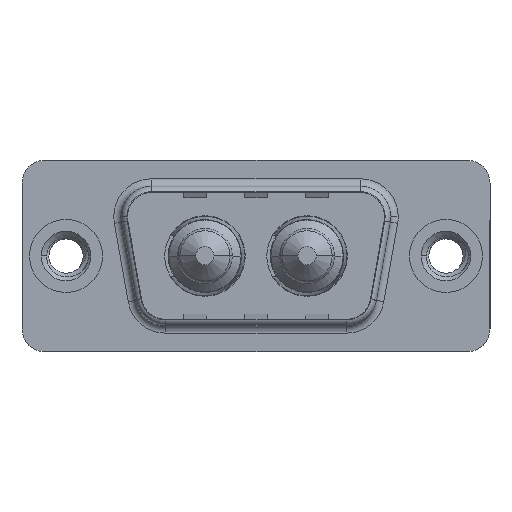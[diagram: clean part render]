
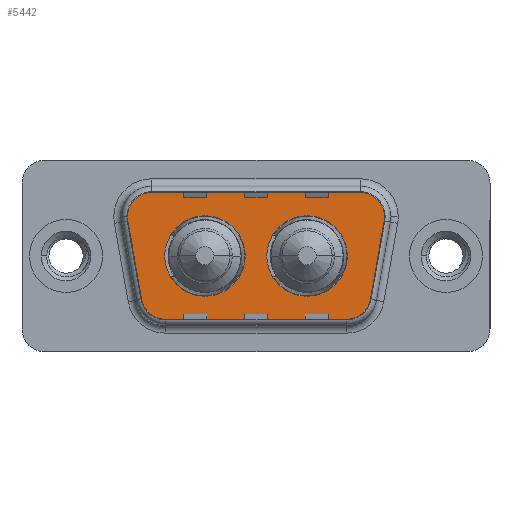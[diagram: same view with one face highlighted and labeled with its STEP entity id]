
A CAD part, top view. The second image highlights one B-rep face of the part: STEP entity #5442.
In plain terms, the highlighted planar face has unit normal (0, 0, 1).
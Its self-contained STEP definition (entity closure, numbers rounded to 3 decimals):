
#39 = CARTESIAN_POINT ( 'NONE',  ( 11.79, 0., 0. ) ) ;
#186 = CARTESIAN_POINT ( 'NONE',  ( 3.466, 2.553, 0. ) ) ;
#323 = EDGE_CURVE ( 'NONE', #8143, #1185, #8012, .T. ) ;
#445 = CARTESIAN_POINT ( 'NONE',  ( 9.14, 0., 0. ) ) ;
#573 = DIRECTION ( 'NONE',  ( 1., 0., 0. ) ) ;
#593 = DIRECTION ( 'NONE',  ( 1., 0., 0. ) ) ;
#618 = DIRECTION ( 'NONE',  ( 1., 0., 0. ) ) ;
#654 = ORIENTED_EDGE ( 'NONE', *, *, #10079, .T. ) ;
#701 = VERTEX_POINT ( 'NONE', #6546 ) ;
#767 = CARTESIAN_POINT ( 'NONE',  ( 21.534, 2.553, 0. ) ) ;
#799 = CIRCLE ( 'NONE', #5250, 2. ) ;
#1023 = EDGE_CURVE ( 'NONE', #1185, #701, #5825, .T. ) ;
#1087 = AXIS2_PLACEMENT_3D ( 'NONE', #2434, #7390, #7545 ) ;
#1137 = EDGE_CURVE ( 'NONE', #2600, #4111, #9660, .T. ) ;
#1185 = VERTEX_POINT ( 'NONE', #8233 ) ;
#1214 = CIRCLE ( 'NONE', #4423, 2.65 ) ;
#1359 = DIRECTION ( 'NONE',  ( 1., 0., 0. ) ) ;
#1370 = AXIS2_PLACEMENT_3D ( 'NONE', #445, #6747, #1359 ) ;
#1387 = FACE_OUTER_BOUND ( 'NONE', #9283, .T. ) ;
#1562 = CARTESIAN_POINT ( 'NONE',  ( 6.49, 0., 0. ) ) ;
#1762 = EDGE_CURVE ( 'NONE', #6806, #3516, #7042, .T. ) ;
#1924 = CARTESIAN_POINT ( 'NONE',  ( 6.459, -4.9, 0. ) ) ;
#2020 = CARTESIAN_POINT ( 'NONE',  ( 4.489, -3.247, 0. ) ) ;
#2040 = CARTESIAN_POINT ( 'NONE',  ( 19.564, 2.9, 0. ) ) ;
#2048 = ORIENTED_EDGE ( 'NONE', *, *, #5889, .T. ) ;
#2051 = DIRECTION ( 'NONE',  ( 0.174, 0.985, 0. ) ) ;
#2434 = CARTESIAN_POINT ( 'NONE',  ( 15.86, 0., 0. ) ) ;
#2600 = VERTEX_POINT ( 'NONE', #10249 ) ;
#2691 = CARTESIAN_POINT ( 'NONE',  ( 18.541, -2.9, 0. ) ) ;
#2757 = DIRECTION ( 'NONE',  ( 0., 0., 1. ) ) ;
#2824 = ORIENTED_EDGE ( 'NONE', *, *, #1023, .T. ) ;
#2886 = ORIENTED_EDGE ( 'NONE', *, *, #6129, .T. ) ;
#2941 = DIRECTION ( 'NONE',  ( 0., 0., 1. ) ) ;
#3012 = CARTESIAN_POINT ( 'NONE',  ( 19.564, 2.9, 0. ) ) ;
#3511 = EDGE_CURVE ( 'NONE', #8292, #8143, #6203, .T. ) ;
#3516 = VERTEX_POINT ( 'NONE', #2020 ) ;
#3623 = DIRECTION ( 'NONE',  ( 1., 0., 0. ) ) ;
#3687 = ORIENTED_EDGE ( 'NONE', *, *, #1137, .F. ) ;
#3717 = DIRECTION ( 'NONE',  ( 0., 0., 1. ) ) ;
#3773 = ORIENTED_EDGE ( 'NONE', *, *, #10854, .T. ) ;
#3774 = VERTEX_POINT ( 'NONE', #9146 ) ;
#4111 = VERTEX_POINT ( 'NONE', #5278 ) ;
#4423 = AXIS2_PLACEMENT_3D ( 'NONE', #11185, #5972, #573 ) ;
#4465 = DIRECTION ( 'NONE',  ( -1., 0., 0. ) ) ;
#4550 = CARTESIAN_POINT ( 'NONE',  ( 5.436, 4.9, 0. ) ) ;
#4733 = CARTESIAN_POINT ( 'NONE',  ( 21.534, 2.553, 0. ) ) ;
#4785 = LINE ( 'NONE', #4550, #11472 ) ;
#4884 = VERTEX_POINT ( 'NONE', #39 ) ;
#5074 = EDGE_CURVE ( 'NONE', #4111, #2600, #10941, .T. ) ;
#5084 = ORIENTED_EDGE ( 'NONE', *, *, #11024, .F. ) ;
#5250 = AXIS2_PLACEMENT_3D ( 'NONE', #8092, #2757, #8964 ) ;
#5270 = AXIS2_PLACEMENT_3D ( 'NONE', #8267, #2941, #9139 ) ;
#5278 = CARTESIAN_POINT ( 'NONE',  ( 13.21, 0., 0. ) ) ;
#5442 = ADVANCED_FACE ( 'NONE', ( #7924, #8208, #1387 ), #11511, .T. ) ;
#5550 = AXIS2_PLACEMENT_3D ( 'NONE', #3012, #6910, #6583 ) ;
#5825 = CIRCLE ( 'NONE', #5550, 2. ) ;
#5889 = EDGE_CURVE ( 'NONE', #3774, #6806, #6460, .T. ) ;
#5972 = DIRECTION ( 'NONE',  ( 0., 0., 1. ) ) ;
#5996 = DIRECTION ( 'NONE',  ( 0., 0., 1. ) ) ;
#6021 = DIRECTION ( 'NONE',  ( 0., 0., 1. ) ) ;
#6129 = EDGE_CURVE ( 'NONE', #701, #3774, #4785, .T. ) ;
#6203 = LINE ( 'NONE', #767, #7681 ) ;
#6230 = DIRECTION ( 'NONE',  ( 1., 0., 0. ) ) ;
#6460 = CIRCLE ( 'NONE', #7969, 2. ) ;
#6546 = CARTESIAN_POINT ( 'NONE',  ( 19.564, 4.9, 0. ) ) ;
#6573 = CIRCLE ( 'NONE', #1370, 2.65 ) ;
#6583 = DIRECTION ( 'NONE',  ( -1., 0., 0. ) ) ;
#6747 = DIRECTION ( 'NONE',  ( 0., 0., 1. ) ) ;
#6806 = VERTEX_POINT ( 'NONE', #186 ) ;
#6812 = DIRECTION ( 'NONE',  ( 0.174, -0.985, 0. ) ) ;
#6910 = DIRECTION ( 'NONE',  ( 0., 0., 1. ) ) ;
#6920 = ORIENTED_EDGE ( 'NONE', *, *, #11130, .F. ) ;
#7042 = LINE ( 'NONE', #7776, #11406 ) ;
#7204 = ORIENTED_EDGE ( 'NONE', *, *, #1762, .T. ) ;
#7210 = ORIENTED_EDGE ( 'NONE', *, *, #323, .T. ) ;
#7390 = DIRECTION ( 'NONE',  ( 0., 0., 1. ) ) ;
#7412 = VERTEX_POINT ( 'NONE', #1924 ) ;
#7545 = DIRECTION ( 'NONE',  ( 1., 0., 0. ) ) ;
#7552 = CARTESIAN_POINT ( 'NONE',  ( 20.511, -3.247, 0. ) ) ;
#7681 = VECTOR ( 'NONE', #2051, 1000. ) ;
#7688 = ORIENTED_EDGE ( 'NONE', *, *, #9869, .T. ) ;
#7776 = CARTESIAN_POINT ( 'NONE',  ( 3.466, 2.553, 0. ) ) ;
#7908 = VERTEX_POINT ( 'NONE', #10489 ) ;
#7914 = CARTESIAN_POINT ( 'NONE',  ( 6.459, -4.9, 0. ) ) ;
#7924 = FACE_BOUND ( 'NONE', #10119, .T. ) ;
#7969 = AXIS2_PLACEMENT_3D ( 'NONE', #11234, #6021, #618 ) ;
#8012 = CIRCLE ( 'NONE', #9102, 2. ) ;
#8092 = CARTESIAN_POINT ( 'NONE',  ( 6.459, -2.9, 0. ) ) ;
#8143 = VERTEX_POINT ( 'NONE', #4733 ) ;
#8208 = FACE_BOUND ( 'NONE', #10228, .T. ) ;
#8233 = CARTESIAN_POINT ( 'NONE',  ( 21.564, 2.9, 0. ) ) ;
#8267 = CARTESIAN_POINT ( 'NONE',  ( 15.86, 0., 0. ) ) ;
#8292 = VERTEX_POINT ( 'NONE', #7552 ) ;
#8701 = ORIENTED_EDGE ( 'NONE', *, *, #3511, .T. ) ;
#8903 = DIRECTION ( 'NONE',  ( 0., 0., 1. ) ) ;
#8916 = DIRECTION ( 'NONE',  ( -1., 0., 0. ) ) ;
#8964 = DIRECTION ( 'NONE',  ( -1., 0., 0. ) ) ;
#9102 = AXIS2_PLACEMENT_3D ( 'NONE', #2040, #3717, #8916 ) ;
#9139 = DIRECTION ( 'NONE',  ( 1., 0., 0. ) ) ;
#9146 = CARTESIAN_POINT ( 'NONE',  ( 5.436, 4.9, 0. ) ) ;
#9283 = EDGE_LOOP ( 'NONE', ( #7688, #8701, #7210, #2824, #2886, #2048, #7204, #3773, #654 ) ) ;
#9288 = LINE ( 'NONE', #7914, #11339 ) ;
#9660 = CIRCLE ( 'NONE', #1087, 2.65 ) ;
#9869 = EDGE_CURVE ( 'NONE', #7908, #8292, #10927, .T. ) ;
#10079 = EDGE_CURVE ( 'NONE', #7412, #7908, #9288, .T. ) ;
#10119 = EDGE_LOOP ( 'NONE', ( #3687, #10551 ) ) ;
#10228 = EDGE_LOOP ( 'NONE', ( #5084, #6920 ) ) ;
#10249 = CARTESIAN_POINT ( 'NONE',  ( 18.51, 0., 0. ) ) ;
#10489 = CARTESIAN_POINT ( 'NONE',  ( 18.541, -4.9, 0. ) ) ;
#10551 = ORIENTED_EDGE ( 'NONE', *, *, #5074, .F. ) ;
#10634 = VERTEX_POINT ( 'NONE', #1562 ) ;
#10854 = EDGE_CURVE ( 'NONE', #3516, #7412, #799, .T. ) ;
#10927 = CIRCLE ( 'NONE', #11371, 2. ) ;
#10941 = CIRCLE ( 'NONE', #5270, 2.65 ) ;
#11024 = EDGE_CURVE ( 'NONE', #4884, #10634, #6573, .T. ) ;
#11130 = EDGE_CURVE ( 'NONE', #10634, #4884, #1214, .T. ) ;
#11185 = CARTESIAN_POINT ( 'NONE',  ( 9.14, 0., 0. ) ) ;
#11204 = CARTESIAN_POINT ( 'NONE',  ( 18.541, -2.9, 0. ) ) ;
#11234 = CARTESIAN_POINT ( 'NONE',  ( 5.436, 2.9, 0. ) ) ;
#11339 = VECTOR ( 'NONE', #6230, 1000. ) ;
#11371 = AXIS2_PLACEMENT_3D ( 'NONE', #11204, #5996, #593 ) ;
#11406 = VECTOR ( 'NONE', #6812, 1000. ) ;
#11472 = VECTOR ( 'NONE', #4465, 1000. ) ;
#11476 = AXIS2_PLACEMENT_3D ( 'NONE', #2691, #8903, #3623 ) ;
#11511 = PLANE ( 'NONE',  #11476 ) ;
